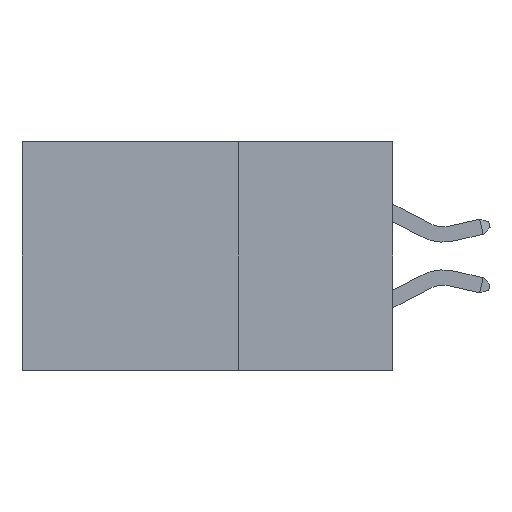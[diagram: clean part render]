
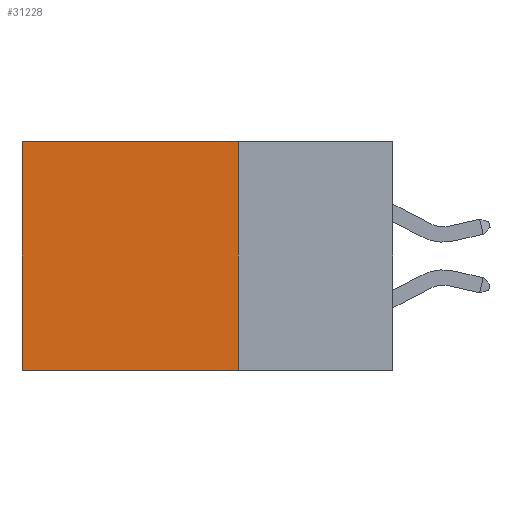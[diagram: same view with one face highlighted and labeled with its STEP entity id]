
A CAD part, left-side view. The second image highlights one B-rep face of the part: STEP entity #31228.
In plain terms, the highlighted planar face has unit normal (-1, 0, 0).
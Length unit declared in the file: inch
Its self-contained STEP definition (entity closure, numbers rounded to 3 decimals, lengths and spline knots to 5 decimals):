
#861 = LINE ( 'NONE', #26508, #4722 ) ;
#1429 = AXIS2_PLACEMENT_3D ( 'NONE', #6296, #17666, #15085 ) ;
#1976 = DIRECTION ( 'NONE',  ( 0., 0., -1. ) ) ;
#3428 = ORIENTED_EDGE ( 'NONE', *, *, #11936, .F. ) ;
#4637 = EDGE_CURVE ( 'NONE', #6089, #27351, #35130, .T. ) ;
#4722 = VECTOR ( 'NONE', #23403, 39.37008 ) ;
#4842 = CARTESIAN_POINT ( 'NONE',  ( 0.2875, 0.6, -0.37 ) ) ;
#4932 = EDGE_LOOP ( 'NONE', ( #26136, #3428, #7144, #24530 ) ) ;
#5097 = EDGE_CURVE ( 'NONE', #6089, #32155, #21237, .T. ) ;
#6089 = VERTEX_POINT ( 'NONE', #16876 ) ;
#6296 = CARTESIAN_POINT ( 'NONE',  ( 0.2875, 0.25, 0. ) ) ;
#7144 = ORIENTED_EDGE ( 'NONE', *, *, #5097, .F. ) ;
#11936 = EDGE_CURVE ( 'NONE', #32155, #13460, #861, .T. ) ;
#13326 = EDGE_CURVE ( 'NONE', #27351, #13460, #28675, .T. ) ;
#13460 = VERTEX_POINT ( 'NONE', #4842 ) ;
#15085 = DIRECTION ( 'NONE',  ( 0., 0., -1. ) ) ;
#16876 = CARTESIAN_POINT ( 'NONE',  ( 0.2875, 0.25, 0. ) ) ;
#17320 = CARTESIAN_POINT ( 'NONE',  ( 0.2875, 0.6, 0. ) ) ;
#17580 = VECTOR ( 'NONE', #28489, 39.37008 ) ;
#17666 = DIRECTION ( 'NONE',  ( 1., 0., 0. ) ) ;
#18350 = CARTESIAN_POINT ( 'NONE',  ( 0.2875, 0.6, 0. ) ) ;
#21237 = LINE ( 'NONE', #26894, #31324 ) ;
#21504 = VECTOR ( 'NONE', #23941, 39.37008 ) ;
#23403 = DIRECTION ( 'NONE',  ( 0., 1., 0. ) ) ;
#23941 = DIRECTION ( 'NONE',  ( 0., 1., 0. ) ) ;
#24530 = ORIENTED_EDGE ( 'NONE', *, *, #4637, .T. ) ;
#24827 = PLANE ( 'NONE',  #1429 ) ;
#26136 = ORIENTED_EDGE ( 'NONE', *, *, #13326, .T. ) ;
#26508 = CARTESIAN_POINT ( 'NONE',  ( 0.2875, 0.25, -0.37 ) ) ;
#26894 = CARTESIAN_POINT ( 'NONE',  ( 0.2875, 0.25, 0. ) ) ;
#27351 = VERTEX_POINT ( 'NONE', #18350 ) ;
#28299 = FACE_OUTER_BOUND ( 'NONE', #4932, .T. ) ;
#28489 = DIRECTION ( 'NONE',  ( 0., 0., -1. ) ) ;
#28675 = LINE ( 'NONE', #17320, #17580 ) ;
#31228 = ADVANCED_FACE ( 'NONE', ( #28299 ), #24827, .F. ) ;
#31324 = VECTOR ( 'NONE', #1976, 39.37008 ) ;
#32155 = VERTEX_POINT ( 'NONE', #34240 ) ;
#32376 = CARTESIAN_POINT ( 'NONE',  ( 0.2875, 0.25, 0. ) ) ;
#34240 = CARTESIAN_POINT ( 'NONE',  ( 0.2875, 0.25, -0.37 ) ) ;
#35130 = LINE ( 'NONE', #32376, #21504 ) ;
